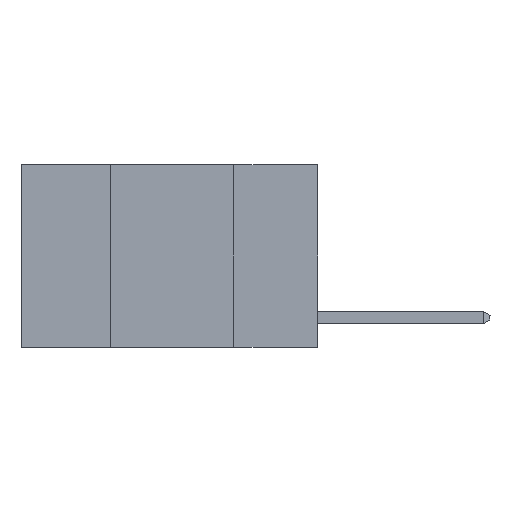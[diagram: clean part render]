
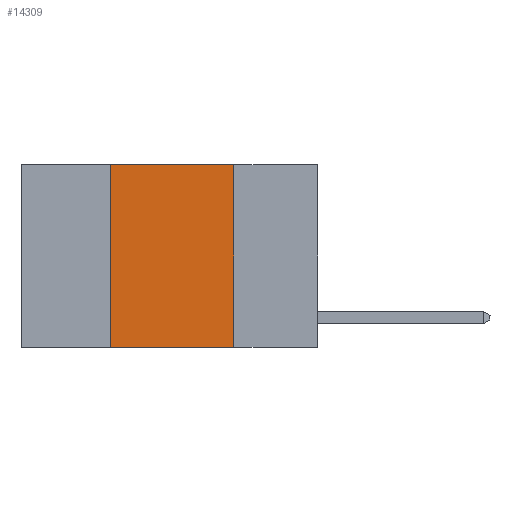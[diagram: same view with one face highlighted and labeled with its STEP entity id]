
A CAD part, left-side view. The second image highlights one B-rep face of the part: STEP entity #14309.
In plain terms, the highlighted planar face has unit normal (-1, 0, 0).
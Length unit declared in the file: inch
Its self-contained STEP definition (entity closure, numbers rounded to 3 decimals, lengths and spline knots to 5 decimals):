
#784 = PLANE ( 'NONE',  #10206 ) ;
#1284 = LINE ( 'NONE', #6131, #17341 ) ;
#1563 = LINE ( 'NONE', #12170, #8180 ) ;
#2299 = VERTEX_POINT ( 'NONE', #9643 ) ;
#2577 = EDGE_CURVE ( 'NONE', #2299, #6069, #17863, .T. ) ;
#2835 = DIRECTION ( 'NONE',  ( 1., 0., 0. ) ) ;
#4465 = CARTESIAN_POINT ( 'NONE',  ( 0., 0.42, 0. ) ) ;
#4535 = DIRECTION ( 'NONE',  ( 0., 0., 1. ) ) ;
#4887 = ORIENTED_EDGE ( 'NONE', *, *, #17292, .F. ) ;
#5583 = LINE ( 'NONE', #10283, #7440 ) ;
#6069 = VERTEX_POINT ( 'NONE', #18322 ) ;
#6131 = CARTESIAN_POINT ( 'NONE',  ( 0., 0.42, 0. ) ) ;
#7440 = VECTOR ( 'NONE', #17525, 39.37008 ) ;
#7540 = ORIENTED_EDGE ( 'NONE', *, *, #12758, .F. ) ;
#7998 = EDGE_CURVE ( 'NONE', #13179, #6069, #1563, .T. ) ;
#8180 = VECTOR ( 'NONE', #14836, 39.37008 ) ;
#9643 = CARTESIAN_POINT ( 'NONE',  ( 0., 0.17, 0. ) ) ;
#10007 = ORIENTED_EDGE ( 'NONE', *, *, #2577, .F. ) ;
#10206 = AXIS2_PLACEMENT_3D ( 'NONE', #12769, #2835, #18063 ) ;
#10283 = CARTESIAN_POINT ( 'NONE',  ( 0., 0.6, 0. ) ) ;
#10414 = DIRECTION ( 'NONE',  ( 0., 0., -1. ) ) ;
#12157 = CARTESIAN_POINT ( 'NONE',  ( 0., 0.17, 0. ) ) ;
#12170 = CARTESIAN_POINT ( 'NONE',  ( 0., 0.6, -0.37 ) ) ;
#12244 = ORIENTED_EDGE ( 'NONE', *, *, #7998, .T. ) ;
#12758 = EDGE_CURVE ( 'NONE', #13179, #17289, #1284, .T. ) ;
#12769 = CARTESIAN_POINT ( 'NONE',  ( 0., 0.6, 0. ) ) ;
#13179 = VERTEX_POINT ( 'NONE', #16571 ) ;
#13428 = EDGE_LOOP ( 'NONE', ( #10007, #4887, #7540, #12244 ) ) ;
#14309 = ADVANCED_FACE ( 'NONE', ( #15717 ), #784, .F. ) ;
#14836 = DIRECTION ( 'NONE',  ( 0., -1., 0. ) ) ;
#15717 = FACE_OUTER_BOUND ( 'NONE', #13428, .T. ) ;
#16571 = CARTESIAN_POINT ( 'NONE',  ( 0., 0.42, -0.37 ) ) ;
#17051 = VECTOR ( 'NONE', #10414, 39.37008 ) ;
#17289 = VERTEX_POINT ( 'NONE', #4465 ) ;
#17292 = EDGE_CURVE ( 'NONE', #17289, #2299, #5583, .T. ) ;
#17341 = VECTOR ( 'NONE', #4535, 39.37008 ) ;
#17525 = DIRECTION ( 'NONE',  ( 0., -1., 0. ) ) ;
#17863 = LINE ( 'NONE', #12157, #17051 ) ;
#18063 = DIRECTION ( 'NONE',  ( 0., 0., -1. ) ) ;
#18322 = CARTESIAN_POINT ( 'NONE',  ( 0., 0.17, -0.37 ) ) ;
